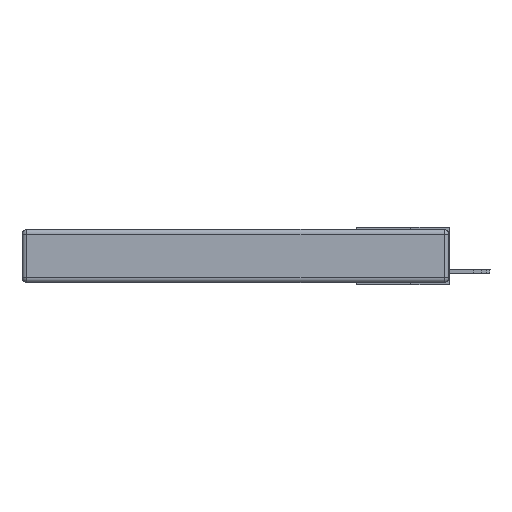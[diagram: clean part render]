
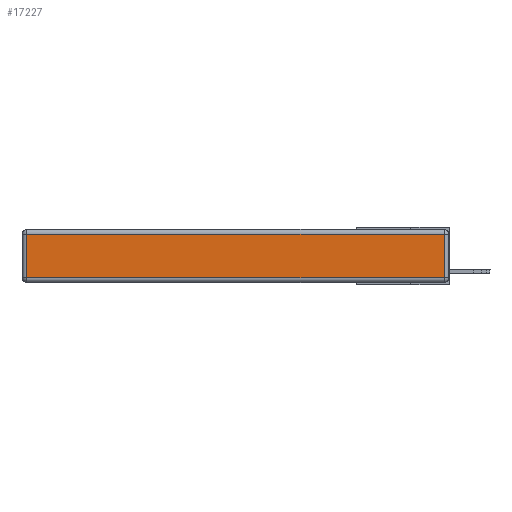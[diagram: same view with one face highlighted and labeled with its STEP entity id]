
A CAD part, left-side view. The second image highlights one B-rep face of the part: STEP entity #17227.
In plain terms, the highlighted planar face has unit normal (-1, 0, 0).
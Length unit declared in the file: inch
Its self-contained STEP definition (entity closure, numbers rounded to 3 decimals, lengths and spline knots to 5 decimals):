
#92 = DIRECTION ( 'NONE',  ( 0., 0., -1. ) ) ;
#1640 = LINE ( 'NONE', #28131, #2340 ) ;
#2027 = ORIENTED_EDGE ( 'NONE', *, *, #20259, .T. ) ;
#2340 = VECTOR ( 'NONE', #8697, 39.37008 ) ;
#4319 = CARTESIAN_POINT ( 'NONE',  ( 0., 0.03, -0.03 ) ) ;
#4525 = CARTESIAN_POINT ( 'NONE',  ( 0., 2.72, -0.313 ) ) ;
#6686 = ORIENTED_EDGE ( 'NONE', *, *, #12214, .T. ) ;
#7369 = DIRECTION ( 'NONE',  ( 0., 1., 0. ) ) ;
#7945 = ORIENTED_EDGE ( 'NONE', *, *, #24140, .T. ) ;
#8616 = EDGE_CURVE ( 'NONE', #16855, #17401, #15361, .T. ) ;
#8697 = DIRECTION ( 'NONE',  ( 0., 0., 1. ) ) ;
#9552 = VECTOR ( 'NONE', #7369, 39.37008 ) ;
#9687 = CARTESIAN_POINT ( 'NONE',  ( 0., 0., -0.313 ) ) ;
#10139 = CARTESIAN_POINT ( 'NONE',  ( 0., 2.75, -0.03 ) ) ;
#12214 = EDGE_CURVE ( 'NONE', #16870, #15986, #20928, .T. ) ;
#12389 = DIRECTION ( 'NONE',  ( -1., 0., 0. ) ) ;
#14322 = DIRECTION ( 'NONE',  ( 0., 0., 1. ) ) ;
#14434 = VECTOR ( 'NONE', #16472, 39.37008 ) ;
#14716 = EDGE_LOOP ( 'NONE', ( #6686, #7945, #23865, #2027 ) ) ;
#15326 = CARTESIAN_POINT ( 'NONE',  ( 0., 0.03, -0.313 ) ) ;
#15361 = LINE ( 'NONE', #10139, #9552 ) ;
#15460 = CARTESIAN_POINT ( 'NONE',  ( 0., 2.72, -0.343 ) ) ;
#15986 = VERTEX_POINT ( 'NONE', #15326 ) ;
#16472 = DIRECTION ( 'NONE',  ( 0., -1., 0. ) ) ;
#16805 = CARTESIAN_POINT ( 'NONE',  ( 0., 0., -0.343 ) ) ;
#16855 = VERTEX_POINT ( 'NONE', #4319 ) ;
#16870 = VERTEX_POINT ( 'NONE', #4525 ) ;
#17227 = ADVANCED_FACE ( 'NONE', ( #19189 ), #25533, .T. ) ;
#17401 = VERTEX_POINT ( 'NONE', #19209 ) ;
#19189 = FACE_OUTER_BOUND ( 'NONE', #14716, .T. ) ;
#19209 = CARTESIAN_POINT ( 'NONE',  ( 0., 2.72, -0.03 ) ) ;
#20259 = EDGE_CURVE ( 'NONE', #17401, #16870, #20716, .T. ) ;
#20716 = LINE ( 'NONE', #15460, #21690 ) ;
#20928 = LINE ( 'NONE', #9687, #14434 ) ;
#21690 = VECTOR ( 'NONE', #92, 39.37008 ) ;
#23865 = ORIENTED_EDGE ( 'NONE', *, *, #8616, .T. ) ;
#24140 = EDGE_CURVE ( 'NONE', #15986, #16855, #1640, .T. ) ;
#25533 = PLANE ( 'NONE',  #27205 ) ;
#27205 = AXIS2_PLACEMENT_3D ( 'NONE', #16805, #12389, #14322 ) ;
#28131 = CARTESIAN_POINT ( 'NONE',  ( 0., 0.03, -0.343 ) ) ;
